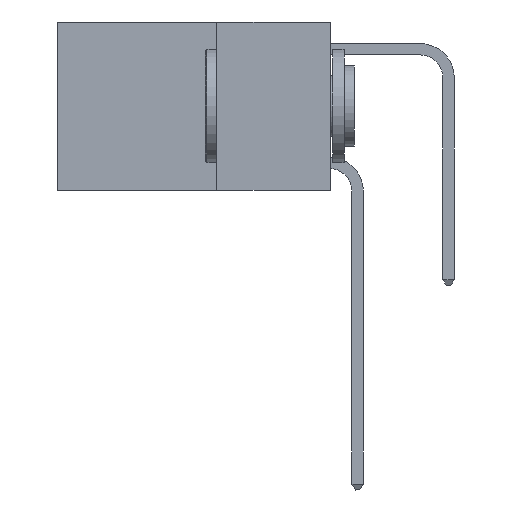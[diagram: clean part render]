
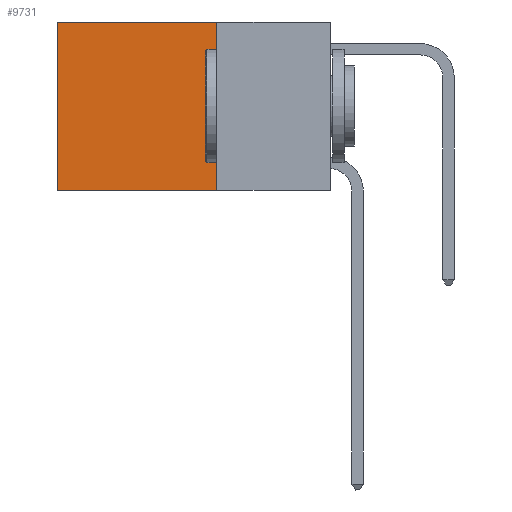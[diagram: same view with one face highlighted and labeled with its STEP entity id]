
A CAD part, left-side view. The second image highlights one B-rep face of the part: STEP entity #9731.
In plain terms, the highlighted planar face has unit normal (-1, 0, 0).
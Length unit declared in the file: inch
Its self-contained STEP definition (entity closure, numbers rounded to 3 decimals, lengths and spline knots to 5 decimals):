
#1176 = ORIENTED_EDGE ( 'NONE', *, *, #27818, .T. ) ;
#2442 = AXIS2_PLACEMENT_3D ( 'NONE', #21178, #16664, #21022 ) ;
#2672 = LINE ( 'NONE', #17821, #25238 ) ;
#3372 = LINE ( 'NONE', #23521, #15823 ) ;
#3380 = CARTESIAN_POINT ( 'NONE',  ( 0.2625, 0.25, 0. ) ) ;
#3983 = CARTESIAN_POINT ( 'NONE',  ( 0.2625, 0.6, 0. ) ) ;
#6011 = ORIENTED_EDGE ( 'NONE', *, *, #6162, .T. ) ;
#6162 = EDGE_CURVE ( 'NONE', #22765, #14706, #11955, .T. ) ;
#6904 = ORIENTED_EDGE ( 'NONE', *, *, #12876, .F. ) ;
#7264 = LINE ( 'NONE', #12427, #8323 ) ;
#8323 = VECTOR ( 'NONE', #22594, 39.37008 ) ;
#9436 = EDGE_LOOP ( 'NONE', ( #6011, #6904, #27634, #1176 ) ) ;
#9731 = ADVANCED_FACE ( 'NONE', ( #11183 ), #13667, .F. ) ;
#11183 = FACE_OUTER_BOUND ( 'NONE', #9436, .T. ) ;
#11955 = LINE ( 'NONE', #3983, #15432 ) ;
#12331 = CARTESIAN_POINT ( 'NONE',  ( 0.2625, 0.6, 0. ) ) ;
#12427 = CARTESIAN_POINT ( 'NONE',  ( 0.2625, 0.25, -0.37 ) ) ;
#12876 = EDGE_CURVE ( 'NONE', #23551, #14706, #7264, .T. ) ;
#13406 = EDGE_CURVE ( 'NONE', #14982, #23551, #3372, .T. ) ;
#13667 = PLANE ( 'NONE',  #2442 ) ;
#13874 = CARTESIAN_POINT ( 'NONE',  ( 0.2625, 0.25, -0.37 ) ) ;
#14116 = DIRECTION ( 'NONE',  ( 0., 0., -1. ) ) ;
#14706 = VERTEX_POINT ( 'NONE', #22391 ) ;
#14982 = VERTEX_POINT ( 'NONE', #3380 ) ;
#15432 = VECTOR ( 'NONE', #14116, 39.37008 ) ;
#15823 = VECTOR ( 'NONE', #28508, 39.37008 ) ;
#16664 = DIRECTION ( 'NONE',  ( 1., 0., 0. ) ) ;
#17821 = CARTESIAN_POINT ( 'NONE',  ( 0.2625, 0.25, 0. ) ) ;
#21022 = DIRECTION ( 'NONE',  ( 0., 0., -1. ) ) ;
#21178 = CARTESIAN_POINT ( 'NONE',  ( 0.2625, 0.25, 0. ) ) ;
#22391 = CARTESIAN_POINT ( 'NONE',  ( 0.2625, 0.6, -0.37 ) ) ;
#22594 = DIRECTION ( 'NONE',  ( 0., 1., 0. ) ) ;
#22765 = VERTEX_POINT ( 'NONE', #12331 ) ;
#23521 = CARTESIAN_POINT ( 'NONE',  ( 0.2625, 0.25, 0. ) ) ;
#23551 = VERTEX_POINT ( 'NONE', #13874 ) ;
#25238 = VECTOR ( 'NONE', #27809, 39.37008 ) ;
#27634 = ORIENTED_EDGE ( 'NONE', *, *, #13406, .F. ) ;
#27809 = DIRECTION ( 'NONE',  ( 0., 1., 0. ) ) ;
#27818 = EDGE_CURVE ( 'NONE', #14982, #22765, #2672, .T. ) ;
#28508 = DIRECTION ( 'NONE',  ( 0., 0., -1. ) ) ;
